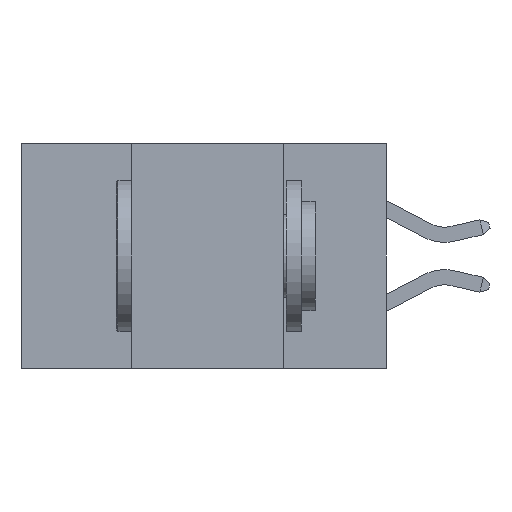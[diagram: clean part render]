
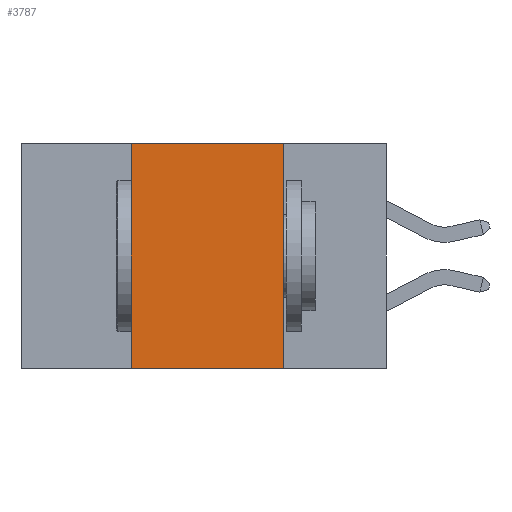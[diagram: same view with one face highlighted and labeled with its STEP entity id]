
A CAD part, left-side view. The second image highlights one B-rep face of the part: STEP entity #3787.
In plain terms, the highlighted planar face has unit normal (-1, 0, 0).
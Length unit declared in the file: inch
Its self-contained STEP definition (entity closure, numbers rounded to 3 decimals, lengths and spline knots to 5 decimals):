
#209 = DIRECTION ( 'NONE',  ( 0., 0., -1. ) ) ;
#231 = VERTEX_POINT ( 'NONE', #5383 ) ;
#702 = LINE ( 'NONE', #13777, #14841 ) ;
#877 = CARTESIAN_POINT ( 'NONE',  ( 0., 0.42, -0.37 ) ) ;
#925 = VERTEX_POINT ( 'NONE', #7526 ) ;
#1756 = DIRECTION ( 'NONE',  ( 0., 0., -1. ) ) ;
#1833 = CARTESIAN_POINT ( 'NONE',  ( 0., 0.6, 0. ) ) ;
#1877 = ORIENTED_EDGE ( 'NONE', *, *, #5962, .F. ) ;
#2088 = PLANE ( 'NONE',  #14161 ) ;
#3411 = DIRECTION ( 'NONE',  ( 1., 0., 0. ) ) ;
#3639 = DIRECTION ( 'NONE',  ( 0., -1., 0. ) ) ;
#3787 = ADVANCED_FACE ( 'NONE', ( #14698 ), #2088, .F. ) ;
#4297 = ORIENTED_EDGE ( 'NONE', *, *, #8907, .F. ) ;
#4672 = DIRECTION ( 'NONE',  ( 0., -1., 0. ) ) ;
#4886 = VERTEX_POINT ( 'NONE', #8113 ) ;
#5383 = CARTESIAN_POINT ( 'NONE',  ( 0., 0.17, -0.37 ) ) ;
#5962 = EDGE_CURVE ( 'NONE', #13330, #4886, #702, .T. ) ;
#6104 = CARTESIAN_POINT ( 'NONE',  ( 0., 0.6, -0.37 ) ) ;
#6315 = EDGE_CURVE ( 'NONE', #925, #231, #11260, .T. ) ;
#6475 = CARTESIAN_POINT ( 'NONE',  ( 0., 0.17, -0.37 ) ) ;
#7192 = CARTESIAN_POINT ( 'NONE',  ( 0., 0.42, 0. ) ) ;
#7451 = EDGE_LOOP ( 'NONE', ( #4297, #1877, #16448, #12281 ) ) ;
#7526 = CARTESIAN_POINT ( 'NONE',  ( 0., 0.42, -0.37 ) ) ;
#8113 = CARTESIAN_POINT ( 'NONE',  ( 0., 0.17, 0. ) ) ;
#8501 = DIRECTION ( 'NONE',  ( 0., 0., 1. ) ) ;
#8758 = VECTOR ( 'NONE', #8501, 39.37008 ) ;
#8836 = LINE ( 'NONE', #877, #8758 ) ;
#8907 = EDGE_CURVE ( 'NONE', #4886, #231, #11977, .T. ) ;
#11260 = LINE ( 'NONE', #6104, #11666 ) ;
#11666 = VECTOR ( 'NONE', #3639, 39.37008 ) ;
#11977 = LINE ( 'NONE', #6475, #16582 ) ;
#12281 = ORIENTED_EDGE ( 'NONE', *, *, #6315, .T. ) ;
#12490 = EDGE_CURVE ( 'NONE', #925, #13330, #8836, .T. ) ;
#13330 = VERTEX_POINT ( 'NONE', #7192 ) ;
#13777 = CARTESIAN_POINT ( 'NONE',  ( 0., 0.6, 0. ) ) ;
#14161 = AXIS2_PLACEMENT_3D ( 'NONE', #1833, #3411, #1756 ) ;
#14698 = FACE_OUTER_BOUND ( 'NONE', #7451, .T. ) ;
#14841 = VECTOR ( 'NONE', #4672, 39.37008 ) ;
#16448 = ORIENTED_EDGE ( 'NONE', *, *, #12490, .F. ) ;
#16582 = VECTOR ( 'NONE', #209, 39.37008 ) ;
